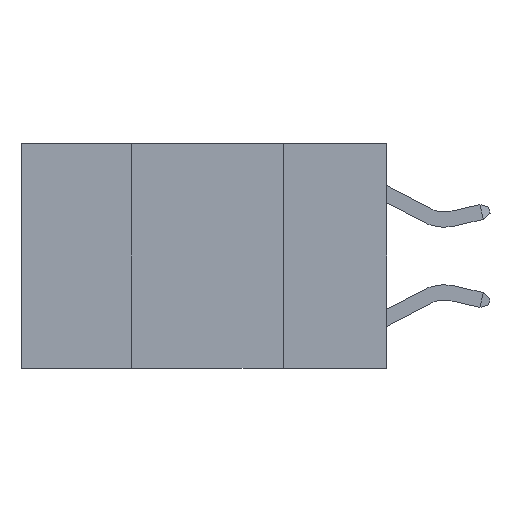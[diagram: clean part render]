
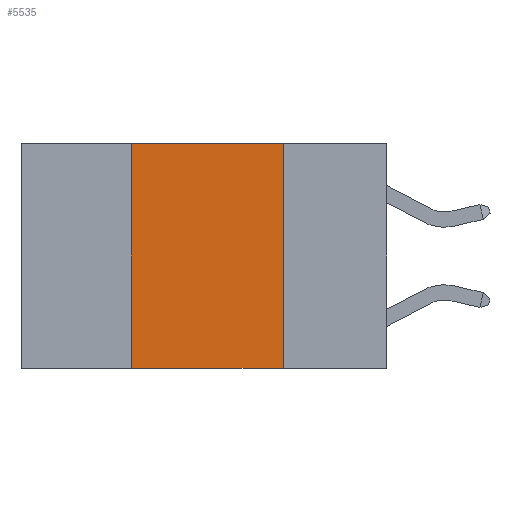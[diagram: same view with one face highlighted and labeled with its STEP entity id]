
A CAD part, left-side view. The second image highlights one B-rep face of the part: STEP entity #5535.
In plain terms, the highlighted planar face has unit normal (-1, 0, 0).
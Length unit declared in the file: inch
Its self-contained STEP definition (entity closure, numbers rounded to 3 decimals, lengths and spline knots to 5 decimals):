
#223 = DIRECTION ( 'NONE',  ( 0., 0., -1. ) ) ;
#1089 = VECTOR ( 'NONE', #15827, 39.37008 ) ;
#1105 = DIRECTION ( 'NONE',  ( 1., 0., 0. ) ) ;
#3241 = ORIENTED_EDGE ( 'NONE', *, *, #10294, .F. ) ;
#4744 = ORIENTED_EDGE ( 'NONE', *, *, #14307, .F. ) ;
#5535 = ADVANCED_FACE ( 'NONE', ( #15836 ), #8755, .F. ) ;
#5764 = CARTESIAN_POINT ( 'NONE',  ( 0., 0.42, 0. ) ) ;
#6494 = CARTESIAN_POINT ( 'NONE',  ( 0., 0.17, 0. ) ) ;
#7278 = VERTEX_POINT ( 'NONE', #11373 ) ;
#8177 = CARTESIAN_POINT ( 'NONE',  ( 0., 0.6, -0.37 ) ) ;
#8755 = PLANE ( 'NONE',  #12075 ) ;
#9410 = CARTESIAN_POINT ( 'NONE',  ( 0., 0.17, 0. ) ) ;
#9621 = DIRECTION ( 'NONE',  ( 0., -1., 0. ) ) ;
#10259 = LINE ( 'NONE', #10573, #13648 ) ;
#10294 = EDGE_CURVE ( 'NONE', #7278, #15628, #10259, .T. ) ;
#10459 = EDGE_CURVE ( 'NONE', #15628, #15392, #18371, .T. ) ;
#10573 = CARTESIAN_POINT ( 'NONE',  ( 0., 0.6, 0. ) ) ;
#10721 = ORIENTED_EDGE ( 'NONE', *, *, #10459, .F. ) ;
#10932 = VECTOR ( 'NONE', #223, 39.37008 ) ;
#11373 = CARTESIAN_POINT ( 'NONE',  ( 0., 0.42, 0. ) ) ;
#11419 = EDGE_CURVE ( 'NONE', #18086, #15392, #16465, .T. ) ;
#11659 = DIRECTION ( 'NONE',  ( 0., 0., -1. ) ) ;
#11873 = CARTESIAN_POINT ( 'NONE',  ( 0., 0.17, -0.37 ) ) ;
#12000 = DIRECTION ( 'NONE',  ( 0., -1., 0. ) ) ;
#12075 = AXIS2_PLACEMENT_3D ( 'NONE', #18597, #1105, #11659 ) ;
#12959 = ORIENTED_EDGE ( 'NONE', *, *, #11419, .T. ) ;
#13648 = VECTOR ( 'NONE', #12000, 39.37008 ) ;
#13840 = EDGE_LOOP ( 'NONE', ( #10721, #3241, #4744, #12959 ) ) ;
#14307 = EDGE_CURVE ( 'NONE', #18086, #7278, #17654, .T. ) ;
#14320 = CARTESIAN_POINT ( 'NONE',  ( 0., 0.42, -0.37 ) ) ;
#15392 = VERTEX_POINT ( 'NONE', #11873 ) ;
#15628 = VERTEX_POINT ( 'NONE', #6494 ) ;
#15827 = DIRECTION ( 'NONE',  ( 0., 0., 1. ) ) ;
#15836 = FACE_OUTER_BOUND ( 'NONE', #13840, .T. ) ;
#16028 = VECTOR ( 'NONE', #9621, 39.37008 ) ;
#16465 = LINE ( 'NONE', #8177, #16028 ) ;
#17654 = LINE ( 'NONE', #5764, #1089 ) ;
#18086 = VERTEX_POINT ( 'NONE', #14320 ) ;
#18371 = LINE ( 'NONE', #9410, #10932 ) ;
#18597 = CARTESIAN_POINT ( 'NONE',  ( 0., 0.6, 0. ) ) ;
